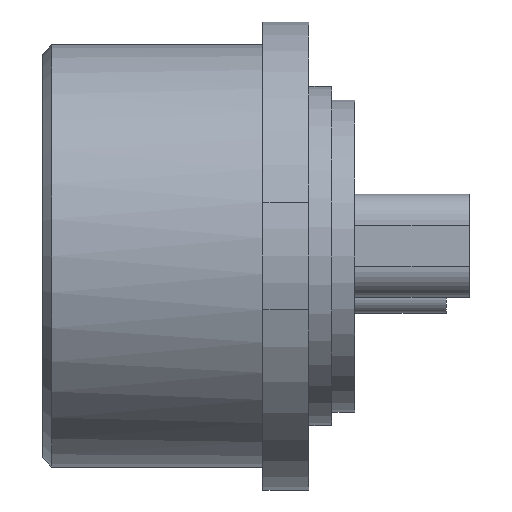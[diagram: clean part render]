
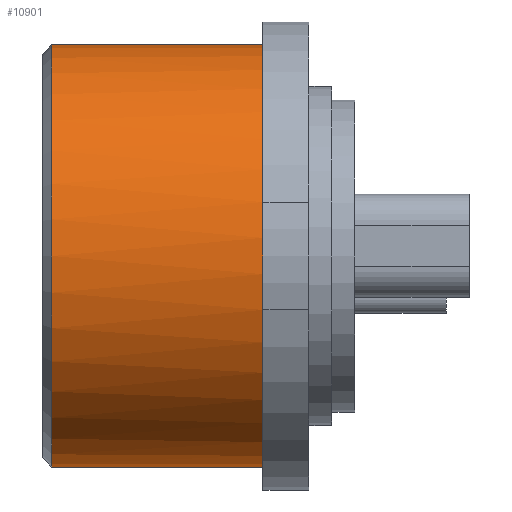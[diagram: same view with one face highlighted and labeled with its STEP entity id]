
A CAD part, left-side view. The second image highlights one B-rep face of the part: STEP entity #10901.
In plain terms, the highlighted cylindrical face has radius 4.6 mm (diameter 9.2 mm), a partial arc.
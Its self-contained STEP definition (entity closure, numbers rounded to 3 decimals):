
#91 = DIRECTION ( 'NONE',  ( 0., 0., -1. ) ) ;
#102 = CARTESIAN_POINT ( 'NONE',  ( -4.675, 1., 0. ) ) ;
#158 = DIRECTION ( 'NONE',  ( 0., 0., 1. ) ) ;
#453 = VERTEX_POINT ( 'NONE', #9877 ) ;
#592 = EDGE_CURVE ( 'NONE', #3124, #998, #7373, .T. ) ;
#625 = DIRECTION ( 'NONE',  ( 0., 1., 0. ) ) ;
#856 = LINE ( 'NONE', #7340, #10866 ) ;
#864 = CARTESIAN_POINT ( 'NONE',  ( -9.122, 1., 1.175 ) ) ;
#998 = VERTEX_POINT ( 'NONE', #5506 ) ;
#1069 = DIRECTION ( 'NONE',  ( 0., -1., 0. ) ) ;
#1375 = ORIENTED_EDGE ( 'NONE', *, *, #10810, .T. ) ;
#2576 = EDGE_CURVE ( 'NONE', #453, #998, #11168, .T. ) ;
#2724 = DIRECTION ( 'NONE',  ( 0., 0., 1. ) ) ;
#2945 = VECTOR ( 'NONE', #625, 1000. ) ;
#3124 = VERTEX_POINT ( 'NONE', #864 ) ;
#3709 = DIRECTION ( 'NONE',  ( 0., 1., 0. ) ) ;
#3718 = EDGE_CURVE ( 'NONE', #453, #8121, #856, .T. ) ;
#3859 = DIRECTION ( 'NONE',  ( 0., 1., 0. ) ) ;
#3969 = DIRECTION ( 'NONE',  ( 0., 1., 0. ) ) ;
#4388 = ORIENTED_EDGE ( 'NONE', *, *, #2576, .T. ) ;
#4593 = CARTESIAN_POINT ( 'NONE',  ( -4.675, 5.6, -4.6 ) ) ;
#4932 = DIRECTION ( 'NONE',  ( 0., 0., 1. ) ) ;
#5093 = CARTESIAN_POINT ( 'NONE',  ( -4.675, 1., 4.6 ) ) ;
#5105 = VERTEX_POINT ( 'NONE', #6404 ) ;
#5506 = CARTESIAN_POINT ( 'NONE',  ( -9.122, 1., -1.175 ) ) ;
#6292 = DIRECTION ( 'NONE',  ( 0., 1., 0. ) ) ;
#6404 = CARTESIAN_POINT ( 'NONE',  ( -4.675, 5.6, 4.6 ) ) ;
#6869 = EDGE_CURVE ( 'NONE', #3124, #7696, #7915, .T. ) ;
#7106 = EDGE_CURVE ( 'NONE', #7696, #5105, #8858, .T. ) ;
#7140 = DIRECTION ( 'NONE',  ( 0., 0., 1. ) ) ;
#7340 = CARTESIAN_POINT ( 'NONE',  ( -4.675, 1., -4.6 ) ) ;
#7373 = CIRCLE ( 'NONE', #10666, 4.6 ) ;
#7422 = CARTESIAN_POINT ( 'NONE',  ( -4.675, 1., 0. ) ) ;
#7631 = AXIS2_PLACEMENT_3D ( 'NONE', #10626, #6292, #7140 ) ;
#7696 = VERTEX_POINT ( 'NONE', #10018 ) ;
#7869 = ORIENTED_EDGE ( 'NONE', *, *, #7106, .T. ) ;
#7915 = CIRCLE ( 'NONE', #9470, 4.6 ) ;
#8121 = VERTEX_POINT ( 'NONE', #4593 ) ;
#8372 = CARTESIAN_POINT ( 'NONE',  ( -4.675, 1., 0. ) ) ;
#8440 = CARTESIAN_POINT ( 'NONE',  ( -4.675, 5.6, 0. ) ) ;
#8640 = ORIENTED_EDGE ( 'NONE', *, *, #6869, .T. ) ;
#8858 = LINE ( 'NONE', #5093, #2945 ) ;
#9201 = CIRCLE ( 'NONE', #11713, 4.6 ) ;
#9470 = AXIS2_PLACEMENT_3D ( 'NONE', #102, #3859, #158 ) ;
#9740 = ORIENTED_EDGE ( 'NONE', *, *, #592, .F. ) ;
#9877 = CARTESIAN_POINT ( 'NONE',  ( -4.675, 1., -4.6 ) ) ;
#10018 = CARTESIAN_POINT ( 'NONE',  ( -4.675, 1., 4.6 ) ) ;
#10567 = FACE_OUTER_BOUND ( 'NONE', #11613, .T. ) ;
#10579 = AXIS2_PLACEMENT_3D ( 'NONE', #8372, #3969, #4932 ) ;
#10626 = CARTESIAN_POINT ( 'NONE',  ( -4.675, 1., 0. ) ) ;
#10666 = AXIS2_PLACEMENT_3D ( 'NONE', #7422, #1069, #91 ) ;
#10810 = EDGE_CURVE ( 'NONE', #5105, #8121, #9201, .T. ) ;
#10866 = VECTOR ( 'NONE', #3709, 1000. ) ;
#10901 = ADVANCED_FACE ( 'NONE', ( #10567 ), #11309, .T. ) ;
#11168 = CIRCLE ( 'NONE', #10579, 4.6 ) ;
#11187 = DIRECTION ( 'NONE',  ( 0., -1., 0. ) ) ;
#11309 = CYLINDRICAL_SURFACE ( 'NONE', #7631, 4.6 ) ;
#11390 = ORIENTED_EDGE ( 'NONE', *, *, #3718, .F. ) ;
#11613 = EDGE_LOOP ( 'NONE', ( #4388, #9740, #8640, #7869, #1375, #11390 ) ) ;
#11713 = AXIS2_PLACEMENT_3D ( 'NONE', #8440, #11187, #2724 ) ;
